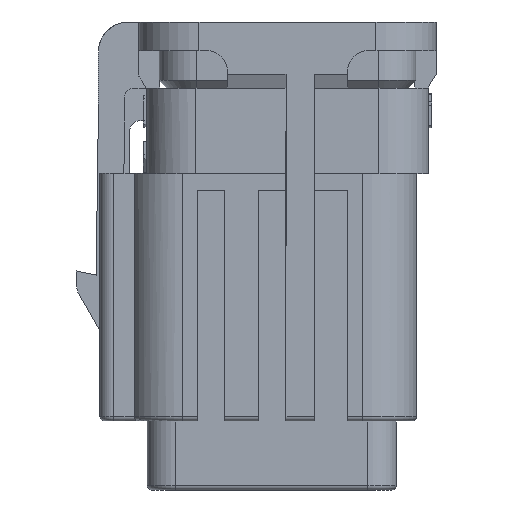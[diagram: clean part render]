
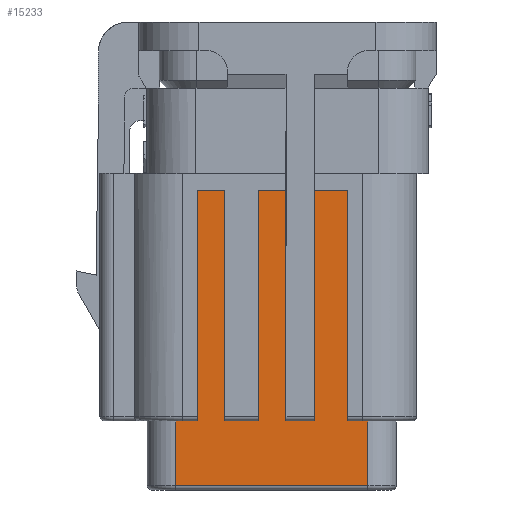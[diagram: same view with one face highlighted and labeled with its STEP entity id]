
A CAD part, left-side view. The second image highlights one B-rep face of the part: STEP entity #15233.
In plain terms, the highlighted planar face has unit normal (-1, 0, 0).
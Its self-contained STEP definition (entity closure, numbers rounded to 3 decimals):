
#52 = LINE ( 'NONE', #231, #8884 ) ;
#191 = CARTESIAN_POINT ( 'NONE',  ( -5.524, 3.508, -5.5 ) ) ;
#231 = CARTESIAN_POINT ( 'NONE',  ( -5.524, -3.842, -5.5 ) ) ;
#373 = EDGE_CURVE ( 'NONE', #17249, #19362, #21493, .T. ) ;
#496 = CARTESIAN_POINT ( 'NONE',  ( -5.524, -3.842, -5.5 ) ) ;
#659 = VERTEX_POINT ( 'NONE', #31256 ) ;
#1021 = VERTEX_POINT ( 'NONE', #27338 ) ;
#1101 = VECTOR ( 'NONE', #26126, 1000. ) ;
#1848 = CARTESIAN_POINT ( 'NONE',  ( -5.524, 2.558, -5.5 ) ) ;
#2204 = CARTESIAN_POINT ( 'NONE',  ( -5.524, 3.508, -5.5 ) ) ;
#2326 = DIRECTION ( 'NONE',  ( 0., -1., 0. ) ) ;
#2361 = CARTESIAN_POINT ( 'NONE',  ( -5.524, -2.067, 2.2 ) ) ;
#2569 = ORIENTED_EDGE ( 'NONE', *, *, #21728, .F. ) ;
#2832 = ORIENTED_EDGE ( 'NONE', *, *, #15494, .F. ) ;
#2883 = VERTEX_POINT ( 'NONE', #2361 ) ;
#3274 = VERTEX_POINT ( 'NONE', #26137 ) ;
#3436 = DIRECTION ( 'NONE',  ( 0., -1., 0. ) ) ;
#3739 = EDGE_CURVE ( 'NONE', #14912, #19362, #4139, .T. ) ;
#3780 = EDGE_CURVE ( 'NONE', #16297, #2883, #18327, .T. ) ;
#4139 = LINE ( 'NONE', #20881, #34426 ) ;
#4192 = DIRECTION ( 'NONE',  ( 0., -1., 0. ) ) ;
#4227 = ORIENTED_EDGE ( 'NONE', *, *, #16236, .T. ) ;
#4551 = CARTESIAN_POINT ( 'NONE',  ( -5.524, 3.508, -7.65 ) ) ;
#5116 = CARTESIAN_POINT ( 'NONE',  ( -5.524, -3.167, -5.5 ) ) ;
#5202 = VERTEX_POINT ( 'NONE', #496 ) ;
#5691 = DIRECTION ( 'NONE',  ( 0., 0., 1. ) ) ;
#6186 = ORIENTED_EDGE ( 'NONE', *, *, #16489, .F. ) ;
#6237 = VERTEX_POINT ( 'NONE', #5116 ) ;
#6375 = EDGE_CURVE ( 'NONE', #5202, #6237, #31734, .T. ) ;
#6912 = CARTESIAN_POINT ( 'NONE',  ( -5.524, -0.217, 2.2 ) ) ;
#6967 = ORIENTED_EDGE ( 'NONE', *, *, #7607, .F. ) ;
#7071 = VERTEX_POINT ( 'NONE', #26524 ) ;
#7105 = LINE ( 'NONE', #4551, #28248 ) ;
#7150 = CARTESIAN_POINT ( 'NONE',  ( -5.524, 3.508, -5.5 ) ) ;
#7596 = ORIENTED_EDGE ( 'NONE', *, *, #29464, .F. ) ;
#7607 = EDGE_CURVE ( 'NONE', #14912, #31714, #17472, .T. ) ;
#7651 = EDGE_CURVE ( 'NONE', #659, #17249, #31800, .T. ) ;
#7659 = CARTESIAN_POINT ( 'NONE',  ( -5.524, 0.933, -5.5 ) ) ;
#7678 = ORIENTED_EDGE ( 'NONE', *, *, #12205, .T. ) ;
#8137 = VERTEX_POINT ( 'NONE', #18281 ) ;
#8547 = VECTOR ( 'NONE', #26168, 1000. ) ;
#8772 = DIRECTION ( 'NONE',  ( 0., 0., 1. ) ) ;
#8884 = VECTOR ( 'NONE', #5691, 1000. ) ;
#8949 = ORIENTED_EDGE ( 'NONE', *, *, #6375, .T. ) ;
#9071 = LINE ( 'NONE', #31243, #32632 ) ;
#9784 = DIRECTION ( 'NONE',  ( 0., 1., 0. ) ) ;
#10987 = ORIENTED_EDGE ( 'NONE', *, *, #373, .F. ) ;
#11190 = VECTOR ( 'NONE', #26556, 1000. ) ;
#11272 = DIRECTION ( 'NONE',  ( 0., 1., 0. ) ) ;
#12205 = EDGE_CURVE ( 'NONE', #24173, #8137, #16497, .T. ) ;
#12294 = CARTESIAN_POINT ( 'NONE',  ( -5.524, 0.933, -5.5 ) ) ;
#13118 = ORIENTED_EDGE ( 'NONE', *, *, #3739, .T. ) ;
#13525 = ORIENTED_EDGE ( 'NONE', *, *, #34836, .F. ) ;
#13562 = CARTESIAN_POINT ( 'NONE',  ( -5.524, -0.217, -5.5 ) ) ;
#13639 = VECTOR ( 'NONE', #11272, 1000. ) ;
#13690 = ORIENTED_EDGE ( 'NONE', *, *, #3780, .F. ) ;
#13874 = FACE_OUTER_BOUND ( 'NONE', #23817, .T. ) ;
#14706 = LINE ( 'NONE', #14886, #1101 ) ;
#14886 = CARTESIAN_POINT ( 'NONE',  ( -5.524, -1.117, -5.5 ) ) ;
#14912 = VERTEX_POINT ( 'NONE', #13562 ) ;
#15041 = VERTEX_POINT ( 'NONE', #20077 ) ;
#15233 = ADVANCED_FACE ( 'NONE', ( #13874 ), #16954, .T. ) ;
#15336 = ORIENTED_EDGE ( 'NONE', *, *, #20363, .T. ) ;
#15494 = EDGE_CURVE ( 'NONE', #2883, #21288, #35389, .T. ) ;
#15783 = DIRECTION ( 'NONE',  ( 0., 0., 1. ) ) ;
#15792 = CARTESIAN_POINT ( 'NONE',  ( -5.524, -3.167, 2.2 ) ) ;
#16222 = VECTOR ( 'NONE', #24478, 1000. ) ;
#16236 = EDGE_CURVE ( 'NONE', #16297, #3274, #32758, .T. ) ;
#16297 = VERTEX_POINT ( 'NONE', #26587 ) ;
#16321 = VECTOR ( 'NONE', #8772, 1000. ) ;
#16489 = EDGE_CURVE ( 'NONE', #21288, #6237, #20223, .T. ) ;
#16497 = LINE ( 'NONE', #27562, #16222 ) ;
#16617 = EDGE_CURVE ( 'NONE', #8137, #15041, #7105, .T. ) ;
#16954 = PLANE ( 'NONE',  #30447 ) ;
#16974 = LINE ( 'NONE', #19706, #16321 ) ;
#16975 = CARTESIAN_POINT ( 'NONE',  ( -5.524, -3.167, 2.2 ) ) ;
#17249 = VERTEX_POINT ( 'NONE', #23706 ) ;
#17472 = LINE ( 'NONE', #6912, #34054 ) ;
#17581 = ORIENTED_EDGE ( 'NONE', *, *, #16617, .T. ) ;
#17820 = VECTOR ( 'NONE', #20575, 1000. ) ;
#18194 = VECTOR ( 'NONE', #15783, 1000. ) ;
#18281 = CARTESIAN_POINT ( 'NONE',  ( -5.524, 2.558, -7.65 ) ) ;
#18327 = LINE ( 'NONE', #32294, #18194 ) ;
#18969 = CARTESIAN_POINT ( 'NONE',  ( -5.524, 3.508, -5.5 ) ) ;
#19290 = ORIENTED_EDGE ( 'NONE', *, *, #7651, .F. ) ;
#19362 = VERTEX_POINT ( 'NONE', #12294 ) ;
#19706 = CARTESIAN_POINT ( 'NONE',  ( -5.524, 1.833, 2.2 ) ) ;
#20037 = CARTESIAN_POINT ( 'NONE',  ( -5.524, -3.167, -5.5 ) ) ;
#20077 = CARTESIAN_POINT ( 'NONE',  ( -5.524, -3.842, -7.65 ) ) ;
#20223 = LINE ( 'NONE', #20037, #17820 ) ;
#20363 = EDGE_CURVE ( 'NONE', #7071, #24173, #32184, .T. ) ;
#20575 = DIRECTION ( 'NONE',  ( 0., 0., -1. ) ) ;
#20881 = CARTESIAN_POINT ( 'NONE',  ( -5.524, 3.508, -5.5 ) ) ;
#21288 = VERTEX_POINT ( 'NONE', #16975 ) ;
#21493 = LINE ( 'NONE', #7659, #11190 ) ;
#21662 = DIRECTION ( 'NONE',  ( 0., 1., 0. ) ) ;
#21728 = EDGE_CURVE ( 'NONE', #7071, #659, #16974, .T. ) ;
#22421 = ORIENTED_EDGE ( 'NONE', *, *, #28484, .T. ) ;
#23646 = VECTOR ( 'NONE', #21662, 1000. ) ;
#23706 = CARTESIAN_POINT ( 'NONE',  ( -5.524, 0.933, 2.2 ) ) ;
#23817 = EDGE_LOOP ( 'NONE', ( #7678, #17581, #22421, #8949, #6186, #2832, #13690, #4227, #13525, #7596, #6967, #13118, #10987, #19290, #2569, #15336 ) ) ;
#24173 = VERTEX_POINT ( 'NONE', #1848 ) ;
#24417 = DIRECTION ( 'NONE',  ( 0., 1., 0. ) ) ;
#24478 = DIRECTION ( 'NONE',  ( 0., 0., -1. ) ) ;
#24767 = DIRECTION ( 'NONE',  ( -1., 0., 0. ) ) ;
#24946 = DIRECTION ( 'NONE',  ( 0., 0., 1. ) ) ;
#25215 = VECTOR ( 'NONE', #2326, 1000. ) ;
#26126 = DIRECTION ( 'NONE',  ( 0., 0., -1. ) ) ;
#26137 = CARTESIAN_POINT ( 'NONE',  ( -5.524, -1.117, -5.5 ) ) ;
#26168 = DIRECTION ( 'NONE',  ( 0., -1., 0. ) ) ;
#26524 = CARTESIAN_POINT ( 'NONE',  ( -5.524, 1.833, -5.5 ) ) ;
#26556 = DIRECTION ( 'NONE',  ( 0., 0., -1. ) ) ;
#26587 = CARTESIAN_POINT ( 'NONE',  ( -5.524, -2.067, -5.5 ) ) ;
#27338 = CARTESIAN_POINT ( 'NONE',  ( -5.524, -1.117, 2.2 ) ) ;
#27562 = CARTESIAN_POINT ( 'NONE',  ( -5.524, 2.558, -5.5 ) ) ;
#28248 = VECTOR ( 'NONE', #4192, 1000. ) ;
#28484 = EDGE_CURVE ( 'NONE', #15041, #5202, #52, .T. ) ;
#28572 = CARTESIAN_POINT ( 'NONE',  ( -5.524, -0.217, 2.2 ) ) ;
#29384 = VECTOR ( 'NONE', #24417, 1000. ) ;
#29464 = EDGE_CURVE ( 'NONE', #31714, #1021, #9071, .T. ) ;
#30447 = AXIS2_PLACEMENT_3D ( 'NONE', #18969, #24767, #24946 ) ;
#31243 = CARTESIAN_POINT ( 'NONE',  ( -5.524, -1.117, 2.2 ) ) ;
#31256 = CARTESIAN_POINT ( 'NONE',  ( -5.524, 1.833, 2.2 ) ) ;
#31714 = VERTEX_POINT ( 'NONE', #28572 ) ;
#31734 = LINE ( 'NONE', #191, #13639 ) ;
#31800 = LINE ( 'NONE', #34334, #8547 ) ;
#32184 = LINE ( 'NONE', #2204, #23646 ) ;
#32294 = CARTESIAN_POINT ( 'NONE',  ( -5.524, -2.067, 2.2 ) ) ;
#32632 = VECTOR ( 'NONE', #3436, 1000. ) ;
#32758 = LINE ( 'NONE', #7150, #29384 ) ;
#34054 = VECTOR ( 'NONE', #34513, 1000. ) ;
#34334 = CARTESIAN_POINT ( 'NONE',  ( -5.524, 0.933, 2.2 ) ) ;
#34426 = VECTOR ( 'NONE', #9784, 1000. ) ;
#34513 = DIRECTION ( 'NONE',  ( 0., 0., 1. ) ) ;
#34836 = EDGE_CURVE ( 'NONE', #1021, #3274, #14706, .T. ) ;
#35389 = LINE ( 'NONE', #15792, #25215 ) ;
